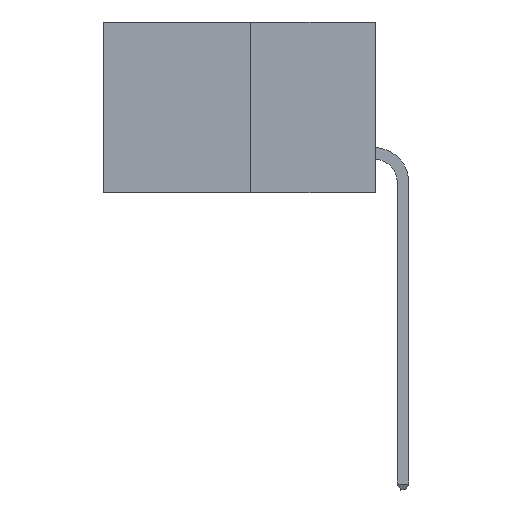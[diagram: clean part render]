
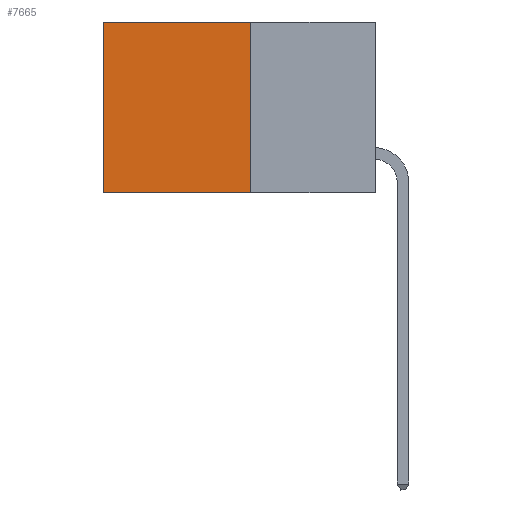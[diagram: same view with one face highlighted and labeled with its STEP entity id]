
A CAD part, left-side view. The second image highlights one B-rep face of the part: STEP entity #7665.
In plain terms, the highlighted planar face has unit normal (-1, 0, 0).
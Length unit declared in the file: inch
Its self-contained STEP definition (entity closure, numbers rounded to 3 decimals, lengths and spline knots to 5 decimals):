
#156 = LINE ( 'NONE', #12987, #12042 ) ;
#372 = EDGE_CURVE ( 'NONE', #9222, #9959, #2406, .T. ) ;
#468 = ORIENTED_EDGE ( 'NONE', *, *, #3344, .F. ) ;
#794 = CARTESIAN_POINT ( 'NONE',  ( 0.277, 0.27, 0. ) ) ;
#1968 = EDGE_LOOP ( 'NONE', ( #2457, #2786, #468, #6331 ) ) ;
#2406 = LINE ( 'NONE', #4025, #10618 ) ;
#2457 = ORIENTED_EDGE ( 'NONE', *, *, #13933, .T. ) ;
#2549 = CARTESIAN_POINT ( 'NONE',  ( 0.277, 0.27, 0. ) ) ;
#2786 = ORIENTED_EDGE ( 'NONE', *, *, #372, .F. ) ;
#3009 = EDGE_CURVE ( 'NONE', #6027, #7154, #11921, .T. ) ;
#3344 = EDGE_CURVE ( 'NONE', #6027, #9222, #6294, .T. ) ;
#3994 = CARTESIAN_POINT ( 'NONE',  ( 0.277, 0.59, -0.37 ) ) ;
#4025 = CARTESIAN_POINT ( 'NONE',  ( 0.277, 0.27, -0.37 ) ) ;
#4541 = CARTESIAN_POINT ( 'NONE',  ( 0.277, 0.27, -0.37 ) ) ;
#5377 = CARTESIAN_POINT ( 'NONE',  ( 0.277, 0.27, -0.37 ) ) ;
#5447 = DIRECTION ( 'NONE',  ( 0., 0., -1. ) ) ;
#5622 = DIRECTION ( 'NONE',  ( 0., 0., -1. ) ) ;
#6027 = VERTEX_POINT ( 'NONE', #2549 ) ;
#6294 = LINE ( 'NONE', #5377, #11581 ) ;
#6302 = DIRECTION ( 'NONE',  ( 0., 1., 0. ) ) ;
#6303 = VECTOR ( 'NONE', #13229, 39.37008 ) ;
#6331 = ORIENTED_EDGE ( 'NONE', *, *, #3009, .T. ) ;
#6374 = CARTESIAN_POINT ( 'NONE',  ( 0.277, 0.59, 0. ) ) ;
#6732 = DIRECTION ( 'NONE',  ( 0., 0., -1. ) ) ;
#7154 = VERTEX_POINT ( 'NONE', #6374 ) ;
#7665 = ADVANCED_FACE ( 'NONE', ( #13143 ), #8830, .F. ) ;
#8830 = PLANE ( 'NONE',  #11144 ) ;
#9222 = VERTEX_POINT ( 'NONE', #13540 ) ;
#9959 = VERTEX_POINT ( 'NONE', #3994 ) ;
#10618 = VECTOR ( 'NONE', #6302, 39.37008 ) ;
#11144 = AXIS2_PLACEMENT_3D ( 'NONE', #4541, #11960, #5622 ) ;
#11581 = VECTOR ( 'NONE', #5447, 39.37008 ) ;
#11921 = LINE ( 'NONE', #794, #6303 ) ;
#11960 = DIRECTION ( 'NONE',  ( 1., 0., 0. ) ) ;
#12042 = VECTOR ( 'NONE', #6732, 39.37008 ) ;
#12987 = CARTESIAN_POINT ( 'NONE',  ( 0.277, 0.59, -0.37 ) ) ;
#13143 = FACE_OUTER_BOUND ( 'NONE', #1968, .T. ) ;
#13229 = DIRECTION ( 'NONE',  ( 0., 1., 0. ) ) ;
#13540 = CARTESIAN_POINT ( 'NONE',  ( 0.277, 0.27, -0.37 ) ) ;
#13933 = EDGE_CURVE ( 'NONE', #7154, #9959, #156, .T. ) ;
